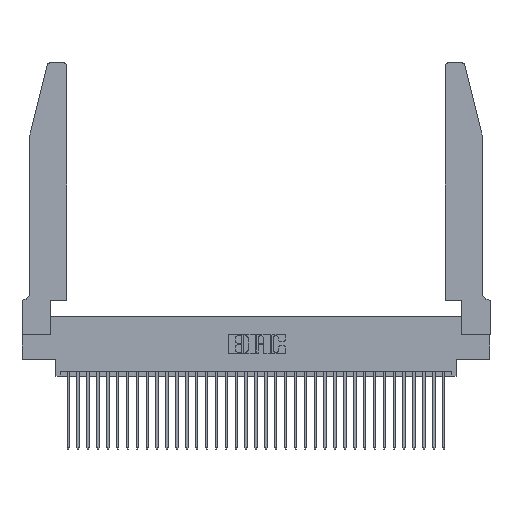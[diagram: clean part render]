
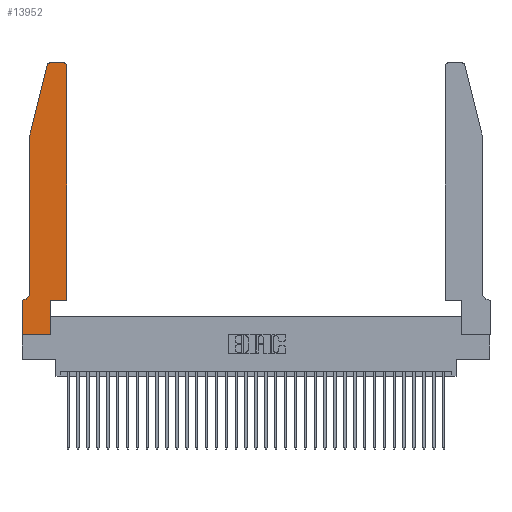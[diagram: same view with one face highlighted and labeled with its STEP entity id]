
A CAD part, top view. The second image highlights one B-rep face of the part: STEP entity #13952.
In plain terms, the highlighted planar face has unit normal (0, 0, 1).
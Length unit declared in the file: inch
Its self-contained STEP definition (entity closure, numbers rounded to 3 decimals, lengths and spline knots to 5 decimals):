
#557 = ORIENTED_EDGE ( 'NONE', *, *, #9371, .T. ) ;
#1163 = CARTESIAN_POINT ( 'NONE',  ( 0., 0., 0.37 ) ) ;
#1369 = VERTEX_POINT ( 'NONE', #29288 ) ;
#1522 = CARTESIAN_POINT ( 'NONE',  ( 0.0055, 0.42, 0.37 ) ) ;
#1578 = CARTESIAN_POINT ( 'NONE',  ( 0.0755, 0.42, 0.37 ) ) ;
#1591 = DIRECTION ( 'NONE',  ( -0.239, -0.971, 0. ) ) ;
#1688 = VECTOR ( 'NONE', #10927, 39.37008 ) ;
#1851 = CARTESIAN_POINT ( 'NONE',  ( 0.0055, 0.35, 0.37 ) ) ;
#2501 = CIRCLE ( 'NONE', #25190, 0.07 ) ;
#2983 = EDGE_LOOP ( 'NONE', ( #22420, #32956, #32160, #16385, #11707, #28325, #7735, #25387, #33049, #12290, #3087, #557 ) ) ;
#3087 = ORIENTED_EDGE ( 'NONE', *, *, #19435, .T. ) ;
#3270 = CIRCLE ( 'NONE', #3361, 0.03 ) ;
#3361 = AXIS2_PLACEMENT_3D ( 'NONE', #12767, #21133, #30313 ) ;
#3521 = CARTESIAN_POINT ( 'NONE',  ( 0.2605, 2.75, 0.37 ) ) ;
#3992 = VERTEX_POINT ( 'NONE', #20445 ) ;
#4070 = DIRECTION ( 'NONE',  ( 1., 0., 0. ) ) ;
#4350 = PLANE ( 'NONE',  #29691 ) ;
#4833 = VERTEX_POINT ( 'NONE', #10393 ) ;
#5118 = DIRECTION ( 'NONE',  ( 0., -1., 0. ) ) ;
#5419 = LINE ( 'NONE', #32825, #19716 ) ;
#5763 = LINE ( 'NONE', #7989, #33095 ) ;
#6451 = EDGE_CURVE ( 'NONE', #31290, #10849, #25961, .T. ) ;
#7567 = CARTESIAN_POINT ( 'NONE',  ( 0., 0., 0.37 ) ) ;
#7735 = ORIENTED_EDGE ( 'NONE', *, *, #25162, .T. ) ;
#7989 = CARTESIAN_POINT ( 'NONE',  ( 0.0755, 2., 0.37 ) ) ;
#9319 = CIRCLE ( 'NONE', #25344, 0.03 ) ;
#9371 = EDGE_CURVE ( 'NONE', #3992, #31290, #3270, .T. ) ;
#10072 = LINE ( 'NONE', #10223, #20433 ) ;
#10223 = CARTESIAN_POINT ( 'NONE',  ( 0.4505, 0.35, 0.37 ) ) ;
#10393 = CARTESIAN_POINT ( 'NONE',  ( 0.0755, 2., 0.37 ) ) ;
#10617 = DIRECTION ( 'NONE',  ( 0., 1., 0. ) ) ;
#10798 = VERTEX_POINT ( 'NONE', #12935 ) ;
#10849 = VERTEX_POINT ( 'NONE', #19034 ) ;
#10927 = DIRECTION ( 'NONE',  ( 0., 1., 0. ) ) ;
#11683 = EDGE_CURVE ( 'NONE', #10849, #19576, #9319, .T. ) ;
#11707 = ORIENTED_EDGE ( 'NONE', *, *, #21527, .T. ) ;
#12290 = ORIENTED_EDGE ( 'NONE', *, *, #25398, .T. ) ;
#12435 = VECTOR ( 'NONE', #30653, 39.37008 ) ;
#12767 = CARTESIAN_POINT ( 'NONE',  ( 0.4205, 2.72, 0.37 ) ) ;
#12935 = CARTESIAN_POINT ( 'NONE',  ( 0.2865, 0.35, 0.37 ) ) ;
#12968 = CARTESIAN_POINT ( 'NONE',  ( 0.4205, 2.75, 0.37 ) ) ;
#12977 = VECTOR ( 'NONE', #1591, 39.37008 ) ;
#13197 = EDGE_CURVE ( 'NONE', #33167, #1369, #15283, .T. ) ;
#13412 = VERTEX_POINT ( 'NONE', #14210 ) ;
#13547 = DIRECTION ( 'NONE',  ( 1., 0., 0. ) ) ;
#13555 = DIRECTION ( 'NONE',  ( -1., 0., 0. ) ) ;
#13924 = VECTOR ( 'NONE', #14612, 39.37008 ) ;
#13952 = ADVANCED_FACE ( 'NONE', ( #18705 ), #4350, .T. ) ;
#14210 = CARTESIAN_POINT ( 'NONE',  ( 0.2865, 0., 0.37 ) ) ;
#14612 = DIRECTION ( 'NONE',  ( -1., 0., 0. ) ) ;
#15056 = VERTEX_POINT ( 'NONE', #1163 ) ;
#15277 = CARTESIAN_POINT ( 'NONE',  ( 0.284, 2.72, 0.37 ) ) ;
#15283 = LINE ( 'NONE', #29576, #26048 ) ;
#15432 = EDGE_CURVE ( 'NONE', #19576, #4833, #22897, .T. ) ;
#16385 = ORIENTED_EDGE ( 'NONE', *, *, #33223, .T. ) ;
#16555 = LINE ( 'NONE', #24046, #1688 ) ;
#18476 = CARTESIAN_POINT ( 'NONE',  ( 0., 0.35, 0.37 ) ) ;
#18705 = FACE_OUTER_BOUND ( 'NONE', #2983, .T. ) ;
#19034 = CARTESIAN_POINT ( 'NONE',  ( 0.284, 2.75, 0.37 ) ) ;
#19435 = EDGE_CURVE ( 'NONE', #24750, #3992, #10072, .T. ) ;
#19576 = VERTEX_POINT ( 'NONE', #30182 ) ;
#19716 = VECTOR ( 'NONE', #5118, 39.37008 ) ;
#20289 = VERTEX_POINT ( 'NONE', #1578 ) ;
#20331 = EDGE_CURVE ( 'NONE', #13412, #10798, #16555, .T. ) ;
#20364 = CARTESIAN_POINT ( 'NONE',  ( 0.4505, 0.35, 0.37 ) ) ;
#20433 = VECTOR ( 'NONE', #10617, 39.37008 ) ;
#20445 = CARTESIAN_POINT ( 'NONE',  ( 0.4505, 2.72, 0.37 ) ) ;
#20703 = DIRECTION ( 'NONE',  ( 0., 0., 1. ) ) ;
#21133 = DIRECTION ( 'NONE',  ( 0., 0., 1. ) ) ;
#21527 = EDGE_CURVE ( 'NONE', #20289, #33167, #2501, .T. ) ;
#22420 = ORIENTED_EDGE ( 'NONE', *, *, #6451, .T. ) ;
#22897 = LINE ( 'NONE', #23683, #12977 ) ;
#23629 = DIRECTION ( 'NONE',  ( 1., 0., 0. ) ) ;
#23683 = CARTESIAN_POINT ( 'NONE',  ( 0.0755, 2., 0.37 ) ) ;
#24046 = CARTESIAN_POINT ( 'NONE',  ( 0.2865, 0.35, 0.37 ) ) ;
#24708 = EDGE_CURVE ( 'NONE', #15056, #13412, #30969, .T. ) ;
#24750 = VERTEX_POINT ( 'NONE', #20364 ) ;
#25162 = EDGE_CURVE ( 'NONE', #1369, #15056, #5419, .T. ) ;
#25190 = AXIS2_PLACEMENT_3D ( 'NONE', #1522, #31931, #34517 ) ;
#25344 = AXIS2_PLACEMENT_3D ( 'NONE', #15277, #20703, #4070 ) ;
#25387 = ORIENTED_EDGE ( 'NONE', *, *, #24708, .T. ) ;
#25398 = EDGE_CURVE ( 'NONE', #10798, #24750, #35313, .T. ) ;
#25961 = LINE ( 'NONE', #3521, #13924 ) ;
#26048 = VECTOR ( 'NONE', #13555, 39.37008 ) ;
#27141 = CARTESIAN_POINT ( 'NONE',  ( 0.4505, 0.35, 0.37 ) ) ;
#27885 = VECTOR ( 'NONE', #13547, 39.37008 ) ;
#28325 = ORIENTED_EDGE ( 'NONE', *, *, #13197, .T. ) ;
#29288 = CARTESIAN_POINT ( 'NONE',  ( 0., 0.35, 0.37 ) ) ;
#29576 = CARTESIAN_POINT ( 'NONE',  ( 0.0755, 0.35, 0.37 ) ) ;
#29691 = AXIS2_PLACEMENT_3D ( 'NONE', #18476, #34531, #23629 ) ;
#29981 = DIRECTION ( 'NONE',  ( 0., -1., 0. ) ) ;
#30182 = CARTESIAN_POINT ( 'NONE',  ( 0.25487, 2.72718, 0.37 ) ) ;
#30313 = DIRECTION ( 'NONE',  ( 1., 0., 0. ) ) ;
#30653 = DIRECTION ( 'NONE',  ( 1., 0., 0. ) ) ;
#30969 = LINE ( 'NONE', #7567, #12435 ) ;
#31290 = VERTEX_POINT ( 'NONE', #12968 ) ;
#31931 = DIRECTION ( 'NONE',  ( 0., 0., -1. ) ) ;
#32160 = ORIENTED_EDGE ( 'NONE', *, *, #15432, .T. ) ;
#32825 = CARTESIAN_POINT ( 'NONE',  ( 0., 0., 0.37 ) ) ;
#32956 = ORIENTED_EDGE ( 'NONE', *, *, #11683, .T. ) ;
#33049 = ORIENTED_EDGE ( 'NONE', *, *, #20331, .T. ) ;
#33095 = VECTOR ( 'NONE', #29981, 39.37008 ) ;
#33167 = VERTEX_POINT ( 'NONE', #1851 ) ;
#33223 = EDGE_CURVE ( 'NONE', #4833, #20289, #5763, .T. ) ;
#34517 = DIRECTION ( 'NONE',  ( -1., 0., 0. ) ) ;
#34531 = DIRECTION ( 'NONE',  ( 0., 0., 1. ) ) ;
#35313 = LINE ( 'NONE', #27141, #27885 ) ;
